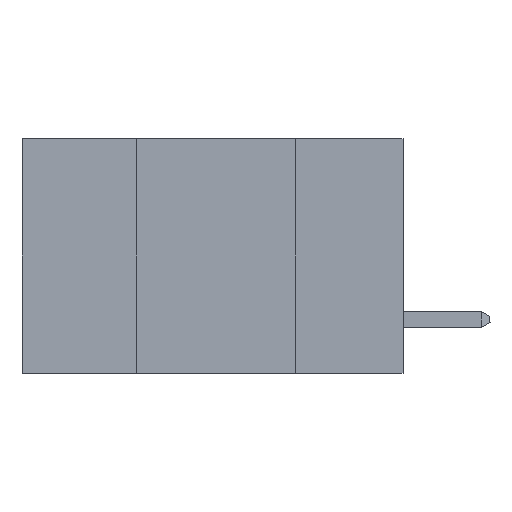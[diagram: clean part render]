
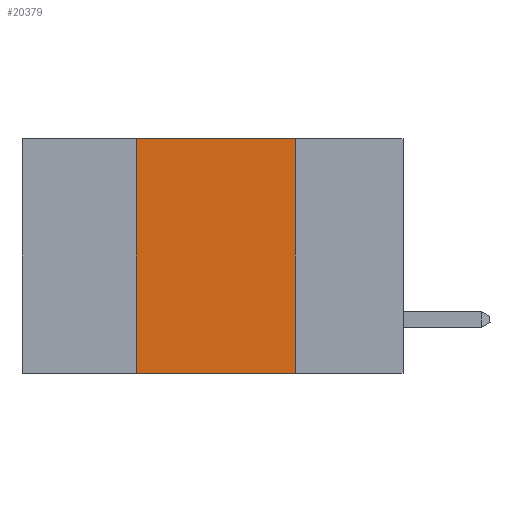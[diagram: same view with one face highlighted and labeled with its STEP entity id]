
A CAD part, left-side view. The second image highlights one B-rep face of the part: STEP entity #20379.
In plain terms, the highlighted planar face has unit normal (-1, 0, 0).
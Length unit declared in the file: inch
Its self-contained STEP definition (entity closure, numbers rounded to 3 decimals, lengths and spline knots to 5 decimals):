
#252 = VERTEX_POINT ( 'NONE', #8831 ) ;
#1720 = ORIENTED_EDGE ( 'NONE', *, *, #22808, .F. ) ;
#1971 = DIRECTION ( 'NONE',  ( 0., -1., 0. ) ) ;
#2819 = CARTESIAN_POINT ( 'NONE',  ( 0., 0.42, 0. ) ) ;
#3399 = VECTOR ( 'NONE', #35202, 39.37008 ) ;
#6992 = VERTEX_POINT ( 'NONE', #14956 ) ;
#7651 = LINE ( 'NONE', #2819, #33728 ) ;
#8425 = ORIENTED_EDGE ( 'NONE', *, *, #11474, .T. ) ;
#8684 = CARTESIAN_POINT ( 'NONE',  ( 0., 0.6, -0.37 ) ) ;
#8831 = CARTESIAN_POINT ( 'NONE',  ( 0., 0.42, 0. ) ) ;
#9172 = FACE_OUTER_BOUND ( 'NONE', #28814, .T. ) ;
#11474 = EDGE_CURVE ( 'NONE', #13355, #6992, #14649, .T. ) ;
#12067 = CARTESIAN_POINT ( 'NONE',  ( 0., 0.17, 0. ) ) ;
#12515 = EDGE_CURVE ( 'NONE', #13355, #252, #7651, .T. ) ;
#13355 = VERTEX_POINT ( 'NONE', #17081 ) ;
#13784 = LINE ( 'NONE', #32922, #24967 ) ;
#14649 = LINE ( 'NONE', #8684, #40719 ) ;
#14956 = CARTESIAN_POINT ( 'NONE',  ( 0., 0.17, -0.37 ) ) ;
#17081 = CARTESIAN_POINT ( 'NONE',  ( 0., 0.42, -0.37 ) ) ;
#17773 = EDGE_CURVE ( 'NONE', #28869, #6992, #29993, .T. ) ;
#17979 = CARTESIAN_POINT ( 'NONE',  ( 0., 0.17, 0. ) ) ;
#19727 = DIRECTION ( 'NONE',  ( 0., -1., 0. ) ) ;
#20063 = AXIS2_PLACEMENT_3D ( 'NONE', #39312, #36724, #26657 ) ;
#20379 = ADVANCED_FACE ( 'NONE', ( #9172 ), #28912, .F. ) ;
#22808 = EDGE_CURVE ( 'NONE', #252, #28869, #13784, .T. ) ;
#24967 = VECTOR ( 'NONE', #19727, 39.37008 ) ;
#26657 = DIRECTION ( 'NONE',  ( 0., 0., -1. ) ) ;
#28814 = EDGE_LOOP ( 'NONE', ( #39543, #1720, #40784, #8425 ) ) ;
#28869 = VERTEX_POINT ( 'NONE', #12067 ) ;
#28912 = PLANE ( 'NONE',  #20063 ) ;
#29993 = LINE ( 'NONE', #17979, #3399 ) ;
#32922 = CARTESIAN_POINT ( 'NONE',  ( 0., 0.6, 0. ) ) ;
#33728 = VECTOR ( 'NONE', #42653, 39.37008 ) ;
#35202 = DIRECTION ( 'NONE',  ( 0., 0., -1. ) ) ;
#36724 = DIRECTION ( 'NONE',  ( 1., 0., 0. ) ) ;
#39312 = CARTESIAN_POINT ( 'NONE',  ( 0., 0.6, 0. ) ) ;
#39543 = ORIENTED_EDGE ( 'NONE', *, *, #17773, .F. ) ;
#40719 = VECTOR ( 'NONE', #1971, 39.37008 ) ;
#40784 = ORIENTED_EDGE ( 'NONE', *, *, #12515, .F. ) ;
#42653 = DIRECTION ( 'NONE',  ( 0., 0., 1. ) ) ;
